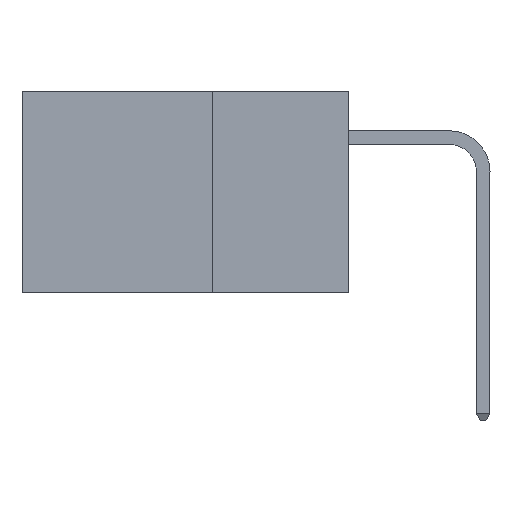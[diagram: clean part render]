
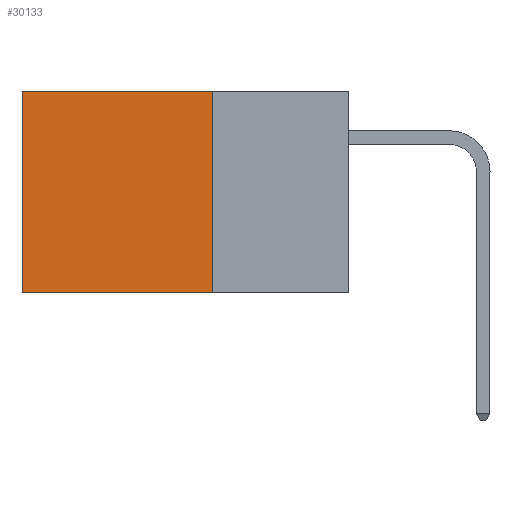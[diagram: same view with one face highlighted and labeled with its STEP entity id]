
A CAD part, left-side view. The second image highlights one B-rep face of the part: STEP entity #30133.
In plain terms, the highlighted planar face has unit normal (-1, 0, 0).
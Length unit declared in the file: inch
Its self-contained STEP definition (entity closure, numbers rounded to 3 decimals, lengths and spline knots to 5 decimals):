
#895 = EDGE_CURVE ( 'NONE', #21740, #22216, #3343, .T. ) ;
#2314 = ORIENTED_EDGE ( 'NONE', *, *, #895, .T. ) ;
#3278 = CARTESIAN_POINT ( 'NONE',  ( 0.2875, 0.25, -0.37 ) ) ;
#3343 = LINE ( 'NONE', #32462, #10274 ) ;
#3747 = LINE ( 'NONE', #18945, #32943 ) ;
#3834 = CARTESIAN_POINT ( 'NONE',  ( 0.2875, 0.6, -0.37 ) ) ;
#6578 = LINE ( 'NONE', #17179, #37433 ) ;
#6958 = VERTEX_POINT ( 'NONE', #3278 ) ;
#7074 = VECTOR ( 'NONE', #33210, 39.37008 ) ;
#8671 = ORIENTED_EDGE ( 'NONE', *, *, #24138, .F. ) ;
#9504 = CARTESIAN_POINT ( 'NONE',  ( 0.2875, 0.25, 0. ) ) ;
#10274 = VECTOR ( 'NONE', #22405, 39.37008 ) ;
#11151 = EDGE_CURVE ( 'NONE', #6958, #32419, #3747, .T. ) ;
#13114 = DIRECTION ( 'NONE',  ( 0., 1., 0. ) ) ;
#14479 = PLANE ( 'NONE',  #28561 ) ;
#17179 = CARTESIAN_POINT ( 'NONE',  ( 0.2875, 0.6, 0. ) ) ;
#18945 = CARTESIAN_POINT ( 'NONE',  ( 0.2875, 0.25, -0.37 ) ) ;
#20394 = DIRECTION ( 'NONE',  ( 0., 0., -1. ) ) ;
#20524 = CARTESIAN_POINT ( 'NONE',  ( 0.2875, 0.6, 0. ) ) ;
#21740 = VERTEX_POINT ( 'NONE', #9504 ) ;
#22216 = VERTEX_POINT ( 'NONE', #20524 ) ;
#22405 = DIRECTION ( 'NONE',  ( 0., 1., 0. ) ) ;
#22858 = EDGE_LOOP ( 'NONE', ( #34945, #34265, #8671, #2314 ) ) ;
#24138 = EDGE_CURVE ( 'NONE', #21740, #6958, #37034, .T. ) ;
#28561 = AXIS2_PLACEMENT_3D ( 'NONE', #34676, #37514, #20394 ) ;
#28723 = DIRECTION ( 'NONE',  ( 0., 0., -1. ) ) ;
#30070 = EDGE_CURVE ( 'NONE', #22216, #32419, #6578, .T. ) ;
#30133 = ADVANCED_FACE ( 'NONE', ( #34772 ), #14479, .F. ) ;
#30358 = CARTESIAN_POINT ( 'NONE',  ( 0.2875, 0.25, 0. ) ) ;
#32419 = VERTEX_POINT ( 'NONE', #3834 ) ;
#32462 = CARTESIAN_POINT ( 'NONE',  ( 0.2875, 0.25, 0. ) ) ;
#32943 = VECTOR ( 'NONE', #13114, 39.37008 ) ;
#33210 = DIRECTION ( 'NONE',  ( 0., 0., -1. ) ) ;
#34265 = ORIENTED_EDGE ( 'NONE', *, *, #11151, .F. ) ;
#34676 = CARTESIAN_POINT ( 'NONE',  ( 0.2875, 0.25, 0. ) ) ;
#34772 = FACE_OUTER_BOUND ( 'NONE', #22858, .T. ) ;
#34945 = ORIENTED_EDGE ( 'NONE', *, *, #30070, .T. ) ;
#37034 = LINE ( 'NONE', #30358, #7074 ) ;
#37433 = VECTOR ( 'NONE', #28723, 39.37008 ) ;
#37514 = DIRECTION ( 'NONE',  ( 1., 0., 0. ) ) ;
